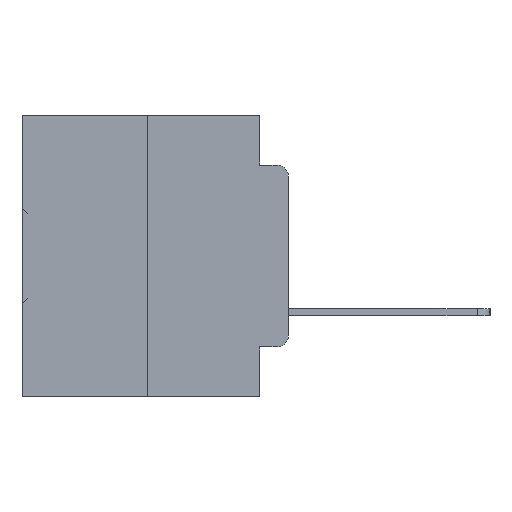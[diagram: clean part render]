
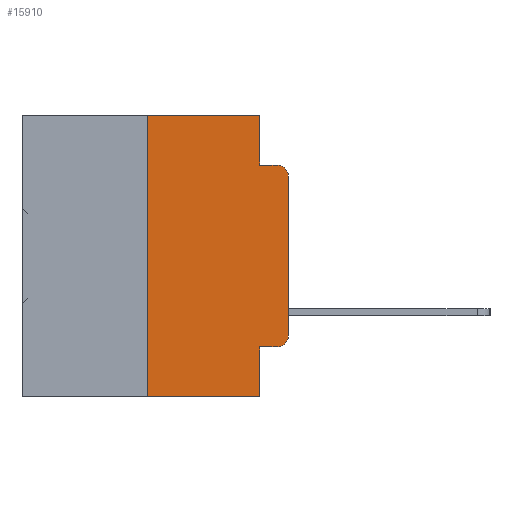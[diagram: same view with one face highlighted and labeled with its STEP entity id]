
A CAD part, left-side view. The second image highlights one B-rep face of the part: STEP entity #15910.
In plain terms, the highlighted planar face has unit normal (-1, 0, 0).
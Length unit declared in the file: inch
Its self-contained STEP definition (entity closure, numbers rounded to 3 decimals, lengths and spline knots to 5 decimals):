
#807 = ORIENTED_EDGE ( 'NONE', *, *, #35191, .F. ) ;
#1777 = VECTOR ( 'NONE', #11328, 39.37008 ) ;
#1818 = CARTESIAN_POINT ( 'NONE',  ( 0., 0.473, 0. ) ) ;
#2663 = ORIENTED_EDGE ( 'NONE', *, *, #26274, .T. ) ;
#3186 = VERTEX_POINT ( 'NONE', #13517 ) ;
#3256 = VERTEX_POINT ( 'NONE', #21116 ) ;
#3431 = CARTESIAN_POINT ( 'NONE',  ( 0., 0.051, -0.0885 ) ) ;
#5320 = LINE ( 'NONE', #20308, #25537 ) ;
#5781 = ORIENTED_EDGE ( 'NONE', *, *, #27452, .T. ) ;
#7284 = CARTESIAN_POINT ( 'NONE',  ( 0., 0.25, -0.5 ) ) ;
#7544 = CARTESIAN_POINT ( 'NONE',  ( 0., 0.02, -0.3915 ) ) ;
#7586 = PLANE ( 'NONE',  #30944 ) ;
#8191 = VERTEX_POINT ( 'NONE', #14309 ) ;
#9301 = VERTEX_POINT ( 'NONE', #24452 ) ;
#9425 = EDGE_CURVE ( 'NONE', #27187, #24356, #17594, .T. ) ;
#9611 = EDGE_CURVE ( 'NONE', #8191, #3186, #32385, .T. ) ;
#10170 = LINE ( 'NONE', #10254, #24724 ) ;
#10254 = CARTESIAN_POINT ( 'NONE',  ( 0., 0.051, -0.4115 ) ) ;
#10373 = DIRECTION ( 'NONE',  ( 0., 0., -1. ) ) ;
#10411 = DIRECTION ( 'NONE',  ( 1., 0., 0. ) ) ;
#11110 = CARTESIAN_POINT ( 'NONE',  ( 0., 0.02, -0.1085 ) ) ;
#11328 = DIRECTION ( 'NONE',  ( 0., 0., -1. ) ) ;
#11717 = VERTEX_POINT ( 'NONE', #7284 ) ;
#11934 = LINE ( 'NONE', #17482, #17515 ) ;
#12125 = LINE ( 'NONE', #18491, #17723 ) ;
#12676 = LINE ( 'NONE', #20377, #19974 ) ;
#12746 = CARTESIAN_POINT ( 'NONE',  ( 0., 0.051, -0.5 ) ) ;
#13517 = CARTESIAN_POINT ( 'NONE',  ( 0., 0., -0.1085 ) ) ;
#13898 = DIRECTION ( 'NONE',  ( 0., 0., -1. ) ) ;
#14309 = CARTESIAN_POINT ( 'NONE',  ( 0., 0., -0.3915 ) ) ;
#14927 = DIRECTION ( 'NONE',  ( 0., 0., 1. ) ) ;
#14942 = DIRECTION ( 'NONE',  ( 0., -1., 0. ) ) ;
#14946 = VECTOR ( 'NONE', #20559, 39.37008 ) ;
#15727 = DIRECTION ( 'NONE',  ( 0., 0., -1. ) ) ;
#15818 = ORIENTED_EDGE ( 'NONE', *, *, #24430, .T. ) ;
#15910 = ADVANCED_FACE ( 'NONE', ( #18194 ), #7586, .F. ) ;
#17080 = CARTESIAN_POINT ( 'NONE',  ( 0., 0.051, 0. ) ) ;
#17482 = CARTESIAN_POINT ( 'NONE',  ( 0., 0.473, 0. ) ) ;
#17515 = VECTOR ( 'NONE', #30990, 39.37008 ) ;
#17562 = CARTESIAN_POINT ( 'NONE',  ( 0., 0., 0. ) ) ;
#17594 = LINE ( 'NONE', #24911, #1777 ) ;
#17723 = VECTOR ( 'NONE', #15727, 39.37008 ) ;
#18006 = VECTOR ( 'NONE', #14927, 39.37008 ) ;
#18194 = FACE_OUTER_BOUND ( 'NONE', #33898, .T. ) ;
#18491 = CARTESIAN_POINT ( 'NONE',  ( 0., 0.051, 0. ) ) ;
#18496 = EDGE_CURVE ( 'NONE', #23104, #24595, #12125, .T. ) ;
#19586 = VERTEX_POINT ( 'NONE', #21247 ) ;
#19948 = CIRCLE ( 'NONE', #31375, 0.02 ) ;
#19974 = VECTOR ( 'NONE', #22996, 39.37008 ) ;
#20308 = CARTESIAN_POINT ( 'NONE',  ( 0., 0.473, -0.5 ) ) ;
#20325 = CARTESIAN_POINT ( 'NONE',  ( 0., 0.25, 0. ) ) ;
#20377 = CARTESIAN_POINT ( 'NONE',  ( 0., 0.051, -0.0885 ) ) ;
#20559 = DIRECTION ( 'NONE',  ( 0., 0., 1. ) ) ;
#21116 = CARTESIAN_POINT ( 'NONE',  ( 0., 0.02, -0.0885 ) ) ;
#21247 = CARTESIAN_POINT ( 'NONE',  ( 0., 0.25, 0. ) ) ;
#22201 = LINE ( 'NONE', #20325, #14946 ) ;
#22996 = DIRECTION ( 'NONE',  ( 0., -1., 0. ) ) ;
#23104 = VERTEX_POINT ( 'NONE', #27966 ) ;
#24356 = VERTEX_POINT ( 'NONE', #3431 ) ;
#24430 = EDGE_CURVE ( 'NONE', #11717, #24595, #5320, .T. ) ;
#24452 = CARTESIAN_POINT ( 'NONE',  ( 0., 0.02, -0.4115 ) ) ;
#24595 = VERTEX_POINT ( 'NONE', #12746 ) ;
#24724 = VECTOR ( 'NONE', #26620, 39.37008 ) ;
#24911 = CARTESIAN_POINT ( 'NONE',  ( 0., 0.051, 0. ) ) ;
#25537 = VECTOR ( 'NONE', #14942, 39.37008 ) ;
#26000 = ORIENTED_EDGE ( 'NONE', *, *, #9611, .T. ) ;
#26274 = EDGE_CURVE ( 'NONE', #23104, #9301, #10170, .T. ) ;
#26372 = CIRCLE ( 'NONE', #31669, 0.02 ) ;
#26620 = DIRECTION ( 'NONE',  ( 0., -1., 0. ) ) ;
#26726 = DIRECTION ( 'NONE',  ( -1., 0., 0. ) ) ;
#27187 = VERTEX_POINT ( 'NONE', #17080 ) ;
#27452 = EDGE_CURVE ( 'NONE', #3186, #3256, #19948, .T. ) ;
#27696 = ORIENTED_EDGE ( 'NONE', *, *, #32037, .F. ) ;
#27966 = CARTESIAN_POINT ( 'NONE',  ( 0., 0.051, -0.4115 ) ) ;
#28549 = ORIENTED_EDGE ( 'NONE', *, *, #35077, .F. ) ;
#29488 = DIRECTION ( 'NONE',  ( 0., 0., -1. ) ) ;
#30172 = DIRECTION ( 'NONE',  ( -1., 0., 0. ) ) ;
#30270 = ORIENTED_EDGE ( 'NONE', *, *, #18496, .F. ) ;
#30944 = AXIS2_PLACEMENT_3D ( 'NONE', #1818, #10411, #29488 ) ;
#30990 = DIRECTION ( 'NONE',  ( 0., -1., 0. ) ) ;
#31208 = EDGE_CURVE ( 'NONE', #9301, #8191, #26372, .T. ) ;
#31375 = AXIS2_PLACEMENT_3D ( 'NONE', #11110, #30172, #13898 ) ;
#31669 = AXIS2_PLACEMENT_3D ( 'NONE', #7544, #26726, #10373 ) ;
#31928 = ORIENTED_EDGE ( 'NONE', *, *, #31208, .T. ) ;
#32037 = EDGE_CURVE ( 'NONE', #24356, #3256, #12676, .T. ) ;
#32385 = LINE ( 'NONE', #17562, #18006 ) ;
#33898 = EDGE_LOOP ( 'NONE', ( #26000, #5781, #27696, #34867, #28549, #807, #15818, #30270, #2663, #31928 ) ) ;
#34867 = ORIENTED_EDGE ( 'NONE', *, *, #9425, .F. ) ;
#35077 = EDGE_CURVE ( 'NONE', #19586, #27187, #11934, .T. ) ;
#35191 = EDGE_CURVE ( 'NONE', #11717, #19586, #22201, .T. ) ;
